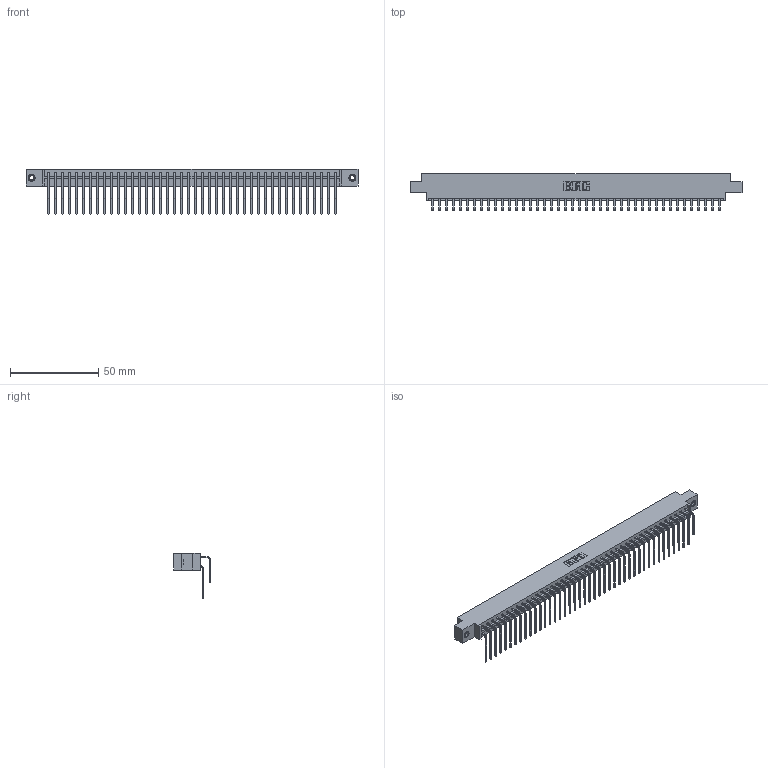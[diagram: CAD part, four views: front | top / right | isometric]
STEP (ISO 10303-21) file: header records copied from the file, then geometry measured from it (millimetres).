
FILE_DESCRIPTION (( 'STEP AP203' ), '1' );
FILE_NAME ('833-084-559-807.STEP', '2020-06-06T02:24:53', ( '' ), ( '' ), 'SwSTEP 2.0', 'SolidWorks 2020', '' );
FILE_SCHEMA (( 'CONFIG_CONTROL_DESIGN' ));
Length unit declared in the file: inch
Products named in the file (5): 833 Part_Offset - .156 Dia - TI; 833-084-559-807; 345-250-001_345-250-005-103; 345-292-001_558 559 Tail - 1; 345-292-001_559 Tail - 2
Assembly tree (87 placements, depth 2):
  833-084-559-807
    833 Part_Offset - .156 Dia - TI
    345-292-001_558 559 Tail - 1  x42
    345-292-001_559 Tail - 2  x42
    345-250-001_345-250-005-103  x2
Bounding box: 187.96 x 20.9 x 25.53 mm (x, y, z)
Volume: 19432.9 mm3; surface area: 25643.2 mm2
Topology: 87 solids, 87 shells, 4714 faces, 13983 edges, 9202 vertices
Faces by surface type: plane 3298, cylinder 1400, cone 12, torus 4
Entity records: 30122 total; most frequent: CARTESIAN_POINT 5028, ORIENTED_EDGE 4906, DIRECTION 4307, EDGE_CURVE 2453, LINE 2265, VECTOR 2265, VERTEX_POINT 1628, AXIS2_PLACEMENT_3D 1021
